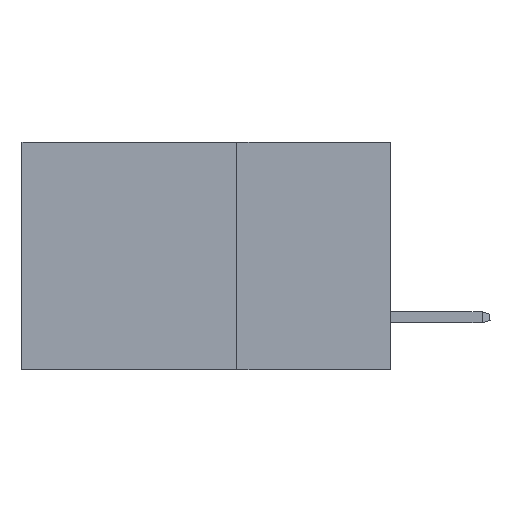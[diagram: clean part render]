
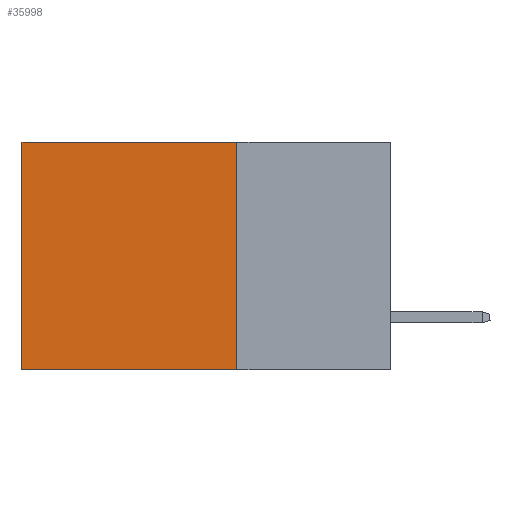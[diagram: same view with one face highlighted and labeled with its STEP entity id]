
A CAD part, left-side view. The second image highlights one B-rep face of the part: STEP entity #35998.
In plain terms, the highlighted planar face has unit normal (-1, 0, 0).
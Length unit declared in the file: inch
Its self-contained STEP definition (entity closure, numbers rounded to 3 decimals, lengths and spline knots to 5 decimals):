
#1808 = EDGE_CURVE ( 'NONE', #22468, #34186, #26410, .T. ) ;
#2708 = CARTESIAN_POINT ( 'NONE',  ( 0.2875, 0.25, 0. ) ) ;
#2870 = VERTEX_POINT ( 'NONE', #32780 ) ;
#3024 = EDGE_CURVE ( 'NONE', #2870, #33080, #4285, .T. ) ;
#4285 = LINE ( 'NONE', #36916, #40958 ) ;
#4308 = CARTESIAN_POINT ( 'NONE',  ( 0.2875, 0.25, 0. ) ) ;
#5448 = VECTOR ( 'NONE', #17380, 39.37008 ) ;
#5680 = ORIENTED_EDGE ( 'NONE', *, *, #11952, .T. ) ;
#7285 = DIRECTION ( 'NONE',  ( 0., 1., 0. ) ) ;
#9880 = EDGE_CURVE ( 'NONE', #22468, #2870, #21241, .T. ) ;
#11932 = CARTESIAN_POINT ( 'NONE',  ( 0.2875, 0.6, 0. ) ) ;
#11952 = EDGE_CURVE ( 'NONE', #34186, #33080, #31504, .T. ) ;
#13322 = CARTESIAN_POINT ( 'NONE',  ( 0.2875, 0.25, 0. ) ) ;
#14473 = ORIENTED_EDGE ( 'NONE', *, *, #9880, .F. ) ;
#14762 = DIRECTION ( 'NONE',  ( 0., 0., -1. ) ) ;
#16830 = DIRECTION ( 'NONE',  ( 1., 0., 0. ) ) ;
#17060 = VECTOR ( 'NONE', #30899, 39.37008 ) ;
#17380 = DIRECTION ( 'NONE',  ( 0., 1., 0. ) ) ;
#21241 = LINE ( 'NONE', #4308, #17060 ) ;
#22468 = VERTEX_POINT ( 'NONE', #2708 ) ;
#26410 = LINE ( 'NONE', #42927, #5448 ) ;
#29977 = DIRECTION ( 'NONE',  ( 0., 0., -1. ) ) ;
#30683 = CARTESIAN_POINT ( 'NONE',  ( 0.2875, 0.6, 0. ) ) ;
#30899 = DIRECTION ( 'NONE',  ( 0., 0., -1. ) ) ;
#31469 = EDGE_LOOP ( 'NONE', ( #5680, #40320, #14473, #40706 ) ) ;
#31504 = LINE ( 'NONE', #11932, #41550 ) ;
#32780 = CARTESIAN_POINT ( 'NONE',  ( 0.2875, 0.25, -0.37 ) ) ;
#33080 = VERTEX_POINT ( 'NONE', #40959 ) ;
#33633 = PLANE ( 'NONE',  #43016 ) ;
#34186 = VERTEX_POINT ( 'NONE', #30683 ) ;
#35998 = ADVANCED_FACE ( 'NONE', ( #42717 ), #33633, .F. ) ;
#36916 = CARTESIAN_POINT ( 'NONE',  ( 0.2875, 0.25, -0.37 ) ) ;
#40320 = ORIENTED_EDGE ( 'NONE', *, *, #3024, .F. ) ;
#40706 = ORIENTED_EDGE ( 'NONE', *, *, #1808, .T. ) ;
#40958 = VECTOR ( 'NONE', #7285, 39.37008 ) ;
#40959 = CARTESIAN_POINT ( 'NONE',  ( 0.2875, 0.6, -0.37 ) ) ;
#41550 = VECTOR ( 'NONE', #14762, 39.37008 ) ;
#42717 = FACE_OUTER_BOUND ( 'NONE', #31469, .T. ) ;
#42927 = CARTESIAN_POINT ( 'NONE',  ( 0.2875, 0.25, 0. ) ) ;
#43016 = AXIS2_PLACEMENT_3D ( 'NONE', #13322, #16830, #29977 ) ;
